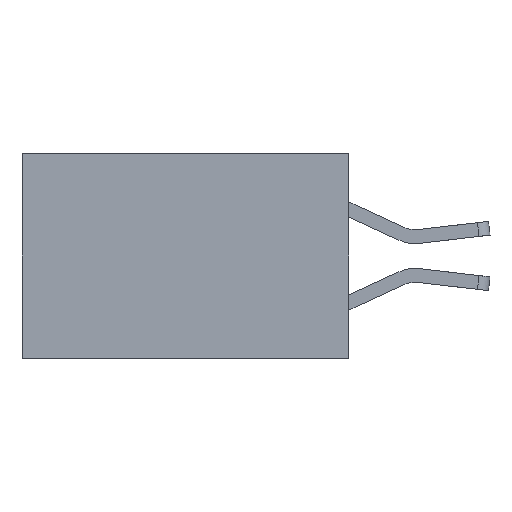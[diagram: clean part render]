
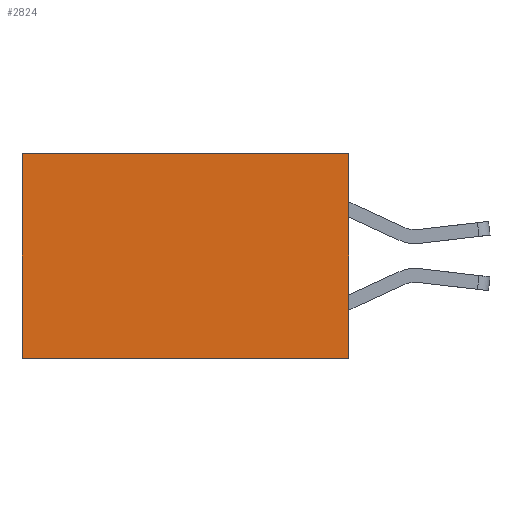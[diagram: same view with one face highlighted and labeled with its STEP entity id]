
A CAD part, left-side view. The second image highlights one B-rep face of the part: STEP entity #2824.
In plain terms, the highlighted planar face has unit normal (-1, 0, 0).
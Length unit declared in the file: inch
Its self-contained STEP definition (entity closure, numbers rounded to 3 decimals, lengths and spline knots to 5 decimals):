
#854 = ORIENTED_EDGE ( 'NONE', *, *, #1916, .F. ) ;
#922 = ORIENTED_EDGE ( 'NONE', *, *, #1069, .T. ) ;
#1069 = EDGE_CURVE ( 'NONE', #5114, #3365, #5427, .T. ) ;
#1297 = CARTESIAN_POINT ( 'NONE',  ( 0.277, 0., -0.37 ) ) ;
#1822 = EDGE_CURVE ( 'NONE', #3571, #7805, #6742, .T. ) ;
#1903 = EDGE_LOOP ( 'NONE', ( #2124, #2874, #854, #922 ) ) ;
#1916 = EDGE_CURVE ( 'NONE', #5114, #3571, #6040, .T. ) ;
#1934 = VECTOR ( 'NONE', #6978, 39.37008 ) ;
#1986 = DIRECTION ( 'NONE',  ( 0., 1., 0. ) ) ;
#2124 = ORIENTED_EDGE ( 'NONE', *, *, #4643, .T. ) ;
#2282 = AXIS2_PLACEMENT_3D ( 'NONE', #5113, #6228, #3672 ) ;
#2552 = FACE_OUTER_BOUND ( 'NONE', #1903, .T. ) ;
#2824 = ADVANCED_FACE ( 'NONE', ( #2552 ), #5698, .F. ) ;
#2874 = ORIENTED_EDGE ( 'NONE', *, *, #1822, .F. ) ;
#3199 = CARTESIAN_POINT ( 'NONE',  ( 0.277, 0.59, -0.37 ) ) ;
#3365 = VERTEX_POINT ( 'NONE', #6315 ) ;
#3451 = VECTOR ( 'NONE', #8176, 39.37008 ) ;
#3515 = CARTESIAN_POINT ( 'NONE',  ( 0.277, 0., 0. ) ) ;
#3571 = VERTEX_POINT ( 'NONE', #1297 ) ;
#3672 = DIRECTION ( 'NONE',  ( 0., 0., -1. ) ) ;
#3716 = CARTESIAN_POINT ( 'NONE',  ( 0.277, 0.59, -0.37 ) ) ;
#4417 = VECTOR ( 'NONE', #6738, 39.37008 ) ;
#4643 = EDGE_CURVE ( 'NONE', #3365, #7805, #8325, .T. ) ;
#5113 = CARTESIAN_POINT ( 'NONE',  ( 0.277, 0., -0.37 ) ) ;
#5114 = VERTEX_POINT ( 'NONE', #5615 ) ;
#5323 = CARTESIAN_POINT ( 'NONE',  ( 0.277, 0., -0.37 ) ) ;
#5427 = LINE ( 'NONE', #3515, #8211 ) ;
#5615 = CARTESIAN_POINT ( 'NONE',  ( 0.277, 0., 0. ) ) ;
#5698 = PLANE ( 'NONE',  #2282 ) ;
#6040 = LINE ( 'NONE', #7599, #4417 ) ;
#6228 = DIRECTION ( 'NONE',  ( 1., 0., 0. ) ) ;
#6315 = CARTESIAN_POINT ( 'NONE',  ( 0.277, 0.59, 0. ) ) ;
#6738 = DIRECTION ( 'NONE',  ( 0., 0., -1. ) ) ;
#6742 = LINE ( 'NONE', #5323, #3451 ) ;
#6978 = DIRECTION ( 'NONE',  ( 0., 0., -1. ) ) ;
#7599 = CARTESIAN_POINT ( 'NONE',  ( 0.277, 0., -0.37 ) ) ;
#7805 = VERTEX_POINT ( 'NONE', #3199 ) ;
#8176 = DIRECTION ( 'NONE',  ( 0., 1., 0. ) ) ;
#8211 = VECTOR ( 'NONE', #1986, 39.37008 ) ;
#8325 = LINE ( 'NONE', #3716, #1934 ) ;
